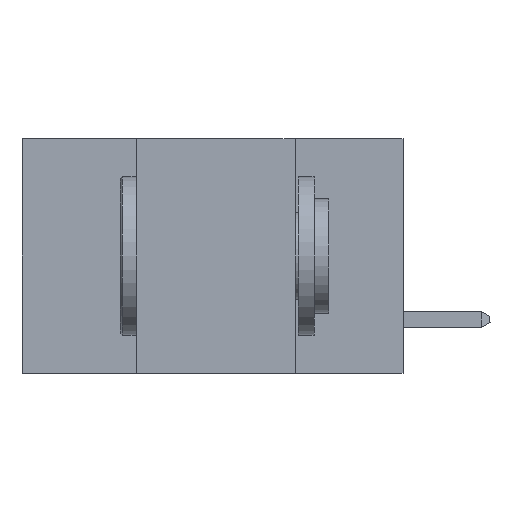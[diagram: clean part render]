
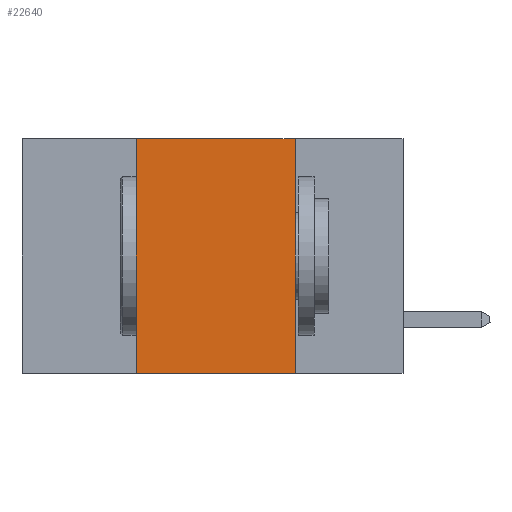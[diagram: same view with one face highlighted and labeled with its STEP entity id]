
A CAD part, left-side view. The second image highlights one B-rep face of the part: STEP entity #22640.
In plain terms, the highlighted planar face has unit normal (-1, 0, 0).
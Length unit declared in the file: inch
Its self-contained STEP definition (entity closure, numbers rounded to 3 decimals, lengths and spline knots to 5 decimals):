
#867 = VERTEX_POINT ( 'NONE', #17355 ) ;
#1270 = CARTESIAN_POINT ( 'NONE',  ( 0., 0.17, 0. ) ) ;
#1504 = LINE ( 'NONE', #18478, #19905 ) ;
#1520 = DIRECTION ( 'NONE',  ( 0., 0., -1. ) ) ;
#1612 = PLANE ( 'NONE',  #20743 ) ;
#1847 = ORIENTED_EDGE ( 'NONE', *, *, #22822, .F. ) ;
#1965 = VECTOR ( 'NONE', #19875, 39.37008 ) ;
#2880 = LINE ( 'NONE', #20778, #23132 ) ;
#2894 = ORIENTED_EDGE ( 'NONE', *, *, #12218, .F. ) ;
#3099 = CARTESIAN_POINT ( 'NONE',  ( 0., 0.42, -0.37 ) ) ;
#5384 = VERTEX_POINT ( 'NONE', #11176 ) ;
#6105 = ORIENTED_EDGE ( 'NONE', *, *, #23512, .T. ) ;
#7058 = EDGE_LOOP ( 'NONE', ( #11272, #2894, #1847, #6105 ) ) ;
#8337 = VECTOR ( 'NONE', #12754, 39.37008 ) ;
#8787 = DIRECTION ( 'NONE',  ( 0., 0., 1. ) ) ;
#11176 = CARTESIAN_POINT ( 'NONE',  ( 0., 0.17, -0.37 ) ) ;
#11272 = ORIENTED_EDGE ( 'NONE', *, *, #18263, .F. ) ;
#12218 = EDGE_CURVE ( 'NONE', #24292, #867, #1504, .T. ) ;
#12515 = DIRECTION ( 'NONE',  ( 0., -1., 0. ) ) ;
#12754 = DIRECTION ( 'NONE',  ( 0., 0., -1. ) ) ;
#13009 = DIRECTION ( 'NONE',  ( 1., 0., 0. ) ) ;
#13221 = CARTESIAN_POINT ( 'NONE',  ( 0., 0.42, 0. ) ) ;
#13661 = VERTEX_POINT ( 'NONE', #3099 ) ;
#17053 = LINE ( 'NONE', #23492, #1965 ) ;
#17355 = CARTESIAN_POINT ( 'NONE',  ( 0., 0.17, 0. ) ) ;
#18263 = EDGE_CURVE ( 'NONE', #867, #5384, #20155, .T. ) ;
#18478 = CARTESIAN_POINT ( 'NONE',  ( 0., 0.6, 0. ) ) ;
#19875 = DIRECTION ( 'NONE',  ( 0., -1., 0. ) ) ;
#19905 = VECTOR ( 'NONE', #12515, 39.37008 ) ;
#20155 = LINE ( 'NONE', #1270, #8337 ) ;
#20743 = AXIS2_PLACEMENT_3D ( 'NONE', #21335, #13009, #1520 ) ;
#20778 = CARTESIAN_POINT ( 'NONE',  ( 0., 0.42, 0. ) ) ;
#21335 = CARTESIAN_POINT ( 'NONE',  ( 0., 0.6, 0. ) ) ;
#22640 = ADVANCED_FACE ( 'NONE', ( #24618 ), #1612, .F. ) ;
#22822 = EDGE_CURVE ( 'NONE', #13661, #24292, #2880, .T. ) ;
#23132 = VECTOR ( 'NONE', #8787, 39.37008 ) ;
#23492 = CARTESIAN_POINT ( 'NONE',  ( 0., 0.6, -0.37 ) ) ;
#23512 = EDGE_CURVE ( 'NONE', #13661, #5384, #17053, .T. ) ;
#24292 = VERTEX_POINT ( 'NONE', #13221 ) ;
#24618 = FACE_OUTER_BOUND ( 'NONE', #7058, .T. ) ;
